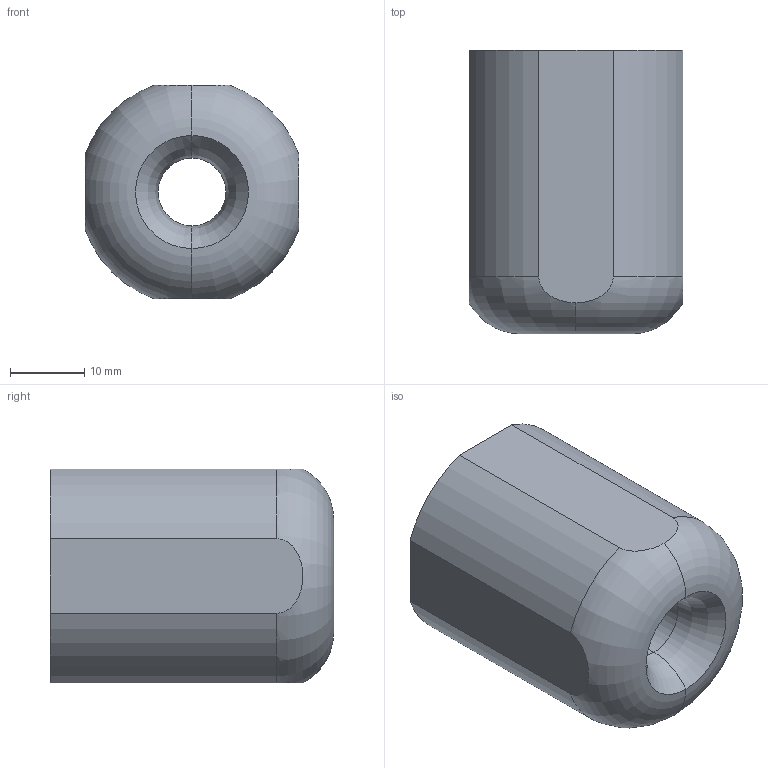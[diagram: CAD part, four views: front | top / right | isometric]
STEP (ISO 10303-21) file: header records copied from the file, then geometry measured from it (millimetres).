
FILE_DESCRIPTION (( 'STEP AP214' ), '1' );
FILE_NAME ('hydra2.0barrel4.STEP', '2013-07-04T02:25:41', ( '' ), ( '' ), 'SwSTEP 2.0', 'SolidWorks 2012', '' );
FILE_SCHEMA (( 'AUTOMOTIVE_DESIGN' ));
Length unit declared in the file: inch
Products named in the file (1): hydra2.0barrel4
Bounding box: 28.76 x 38.1 x 28.76 mm (x, y, z)
Volume: 22702 mm3; surface area: 6037.5 mm2
Topology: 1 solids, 1 shells, 27 faces, 74 edges, 48 vertices
Faces by surface type: cylinder 14, plane 5, torus 4, sphere 4
Entity records: 952 total; most frequent: CARTESIAN_POINT 272, DIRECTION 146, ORIENTED_EDGE 124, EDGE_CURVE 62, AXIS2_PLACEMENT_3D 62, VERTEX_POINT 40, CIRCLE 34, EDGE_LOOP 32
